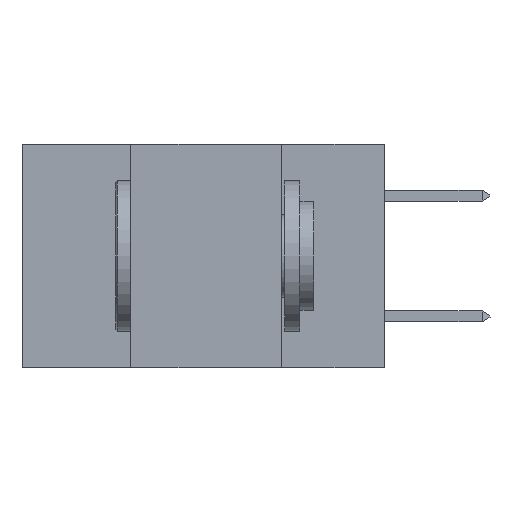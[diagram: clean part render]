
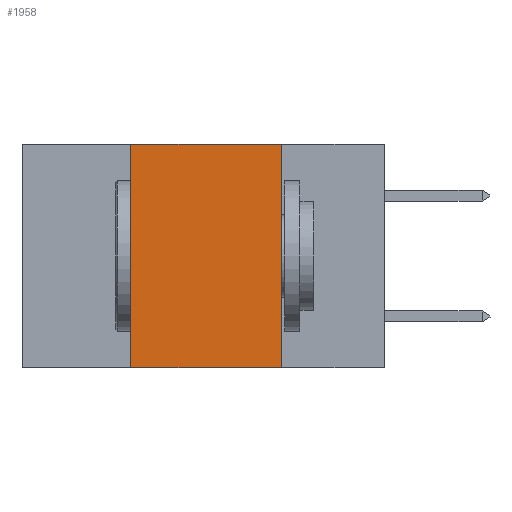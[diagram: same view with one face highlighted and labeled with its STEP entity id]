
A CAD part, left-side view. The second image highlights one B-rep face of the part: STEP entity #1958.
In plain terms, the highlighted planar face has unit normal (-1, 0, 0).
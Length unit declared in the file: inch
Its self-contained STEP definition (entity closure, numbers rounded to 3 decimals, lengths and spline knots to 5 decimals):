
#1269 = ORIENTED_EDGE ( 'NONE', *, *, #3786, .F. ) ;
#1657 = ORIENTED_EDGE ( 'NONE', *, *, #9669, .F. ) ;
#1958 = ADVANCED_FACE ( 'NONE', ( #5618 ), #19030, .F. ) ;
#2602 = CARTESIAN_POINT ( 'NONE',  ( 0., 0.17, 0. ) ) ;
#3424 = VERTEX_POINT ( 'NONE', #2602 ) ;
#3786 = EDGE_CURVE ( 'NONE', #3424, #16730, #22857, .T. ) ;
#3801 = VECTOR ( 'NONE', #10982, 39.37008 ) ;
#4222 = CARTESIAN_POINT ( 'NONE',  ( 0., 0.6, -0.37 ) ) ;
#5216 = ORIENTED_EDGE ( 'NONE', *, *, #13282, .T. ) ;
#5618 = FACE_OUTER_BOUND ( 'NONE', #13878, .T. ) ;
#6844 = EDGE_CURVE ( 'NONE', #15449, #3424, #22801, .T. ) ;
#7115 = CARTESIAN_POINT ( 'NONE',  ( 0., 0.42, 0. ) ) ;
#9669 = EDGE_CURVE ( 'NONE', #12270, #15449, #19698, .T. ) ;
#10373 = DIRECTION ( 'NONE',  ( 1., 0., 0. ) ) ;
#10473 = DIRECTION ( 'NONE',  ( 0., 0., -1. ) ) ;
#10551 = CARTESIAN_POINT ( 'NONE',  ( 0., 0.6, 0. ) ) ;
#10982 = DIRECTION ( 'NONE',  ( 0., 0., -1. ) ) ;
#11117 = CARTESIAN_POINT ( 'NONE',  ( 0., 0.17, 0. ) ) ;
#11158 = AXIS2_PLACEMENT_3D ( 'NONE', #19082, #10373, #10473 ) ;
#11448 = VECTOR ( 'NONE', #20423, 39.37008 ) ;
#12270 = VERTEX_POINT ( 'NONE', #19143 ) ;
#12788 = CARTESIAN_POINT ( 'NONE',  ( 0., 0.17, -0.37 ) ) ;
#13282 = EDGE_CURVE ( 'NONE', #12270, #16730, #15631, .T. ) ;
#13878 = EDGE_LOOP ( 'NONE', ( #1269, #19875, #1657, #5216 ) ) ;
#15449 = VERTEX_POINT ( 'NONE', #18349 ) ;
#15631 = LINE ( 'NONE', #4222, #11448 ) ;
#16730 = VERTEX_POINT ( 'NONE', #12788 ) ;
#18349 = CARTESIAN_POINT ( 'NONE',  ( 0., 0.42, 0. ) ) ;
#18691 = VECTOR ( 'NONE', #22971, 39.37008 ) ;
#19030 = PLANE ( 'NONE',  #11158 ) ;
#19082 = CARTESIAN_POINT ( 'NONE',  ( 0., 0.6, 0. ) ) ;
#19143 = CARTESIAN_POINT ( 'NONE',  ( 0., 0.42, -0.37 ) ) ;
#19636 = DIRECTION ( 'NONE',  ( 0., 0., 1. ) ) ;
#19698 = LINE ( 'NONE', #7115, #20258 ) ;
#19875 = ORIENTED_EDGE ( 'NONE', *, *, #6844, .F. ) ;
#20258 = VECTOR ( 'NONE', #19636, 39.37008 ) ;
#20423 = DIRECTION ( 'NONE',  ( 0., -1., 0. ) ) ;
#22801 = LINE ( 'NONE', #10551, #18691 ) ;
#22857 = LINE ( 'NONE', #11117, #3801 ) ;
#22971 = DIRECTION ( 'NONE',  ( 0., -1., 0. ) ) ;
